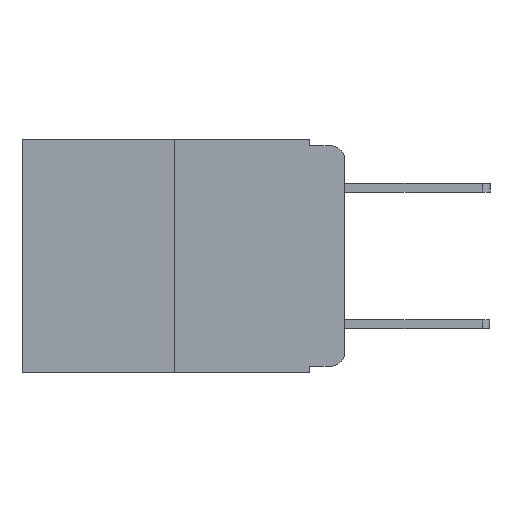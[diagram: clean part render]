
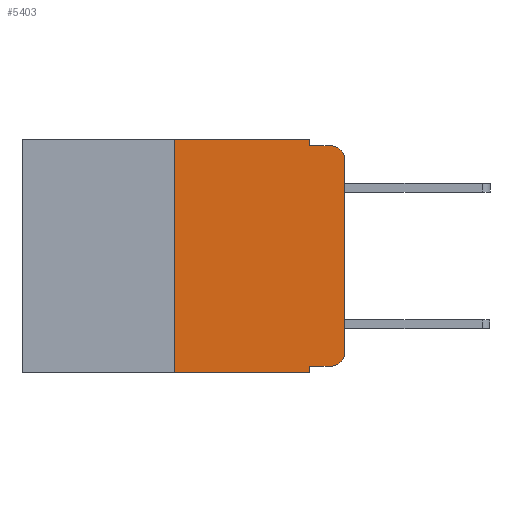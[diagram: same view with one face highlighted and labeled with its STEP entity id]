
A CAD part, left-side view. The second image highlights one B-rep face of the part: STEP entity #5403.
In plain terms, the highlighted planar face has unit normal (-1, 0, 0).
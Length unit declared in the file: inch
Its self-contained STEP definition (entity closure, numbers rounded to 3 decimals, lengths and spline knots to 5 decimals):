
#207 = VERTEX_POINT ( 'NONE', #18770 ) ;
#212 = DIRECTION ( 'NONE',  ( -1., 0., 0. ) ) ;
#791 = VECTOR ( 'NONE', #21845, 39.37008 ) ;
#1542 = VERTEX_POINT ( 'NONE', #19385 ) ;
#1869 = CARTESIAN_POINT ( 'NONE',  ( 0., 0., -0.03 ) ) ;
#1875 = DIRECTION ( 'NONE',  ( 0., 0., -1. ) ) ;
#2363 = VERTEX_POINT ( 'NONE', #11058 ) ;
#2565 = VECTOR ( 'NONE', #14616, 39.37008 ) ;
#2620 = EDGE_CURVE ( 'NONE', #9207, #5391, #18414, .T. ) ;
#2834 = DIRECTION ( 'NONE',  ( -1., 0., 0. ) ) ;
#3682 = DIRECTION ( 'NONE',  ( 0., 0., 1. ) ) ;
#3754 = VERTEX_POINT ( 'NONE', #19878 ) ;
#3795 = CARTESIAN_POINT ( 'NONE',  ( 0., 0.473, -0.343 ) ) ;
#4409 = VERTEX_POINT ( 'NONE', #1869 ) ;
#4679 = DIRECTION ( 'NONE',  ( 1., 0., 0. ) ) ;
#4725 = EDGE_CURVE ( 'NONE', #4409, #1542, #7290, .T. ) ;
#4812 = VECTOR ( 'NONE', #3682, 39.37008 ) ;
#5391 = VERTEX_POINT ( 'NONE', #15419 ) ;
#5403 = ADVANCED_FACE ( 'NONE', ( #17141 ), #22650, .F. ) ;
#5449 = AXIS2_PLACEMENT_3D ( 'NONE', #11180, #212, #12978 ) ;
#5974 = VERTEX_POINT ( 'NONE', #20781 ) ;
#6327 = LINE ( 'NONE', #3795, #2565 ) ;
#6344 = ORIENTED_EDGE ( 'NONE', *, *, #19648, .F. ) ;
#6492 = DIRECTION ( 'NONE',  ( 0., -1., 0. ) ) ;
#6528 = LINE ( 'NONE', #18198, #4812 ) ;
#6679 = ORIENTED_EDGE ( 'NONE', *, *, #6834, .T. ) ;
#6746 = VERTEX_POINT ( 'NONE', #15909 ) ;
#6834 = EDGE_CURVE ( 'NONE', #5974, #5391, #6327, .T. ) ;
#6891 = CARTESIAN_POINT ( 'NONE',  ( 0., 0.051, -0.333 ) ) ;
#6911 = VECTOR ( 'NONE', #1875, 39.37008 ) ;
#7230 = VECTOR ( 'NONE', #8266, 39.37008 ) ;
#7290 = CIRCLE ( 'NONE', #8302, 0.02 ) ;
#7409 = CIRCLE ( 'NONE', #5449, 0.02 ) ;
#7461 = EDGE_CURVE ( 'NONE', #207, #2363, #21291, .T. ) ;
#8266 = DIRECTION ( 'NONE',  ( 0., -1., 0. ) ) ;
#8302 = AXIS2_PLACEMENT_3D ( 'NONE', #13658, #2834, #15533 ) ;
#8913 = CARTESIAN_POINT ( 'NONE',  ( 0., 0.02, -0.333 ) ) ;
#9089 = EDGE_CURVE ( 'NONE', #9207, #21741, #16703, .T. ) ;
#9207 = VERTEX_POINT ( 'NONE', #6891 ) ;
#9549 = ORIENTED_EDGE ( 'NONE', *, *, #2620, .F. ) ;
#9586 = CARTESIAN_POINT ( 'NONE',  ( 0., 0.473, 0. ) ) ;
#10154 = EDGE_LOOP ( 'NONE', ( #18656, #12806, #12876, #14495, #6344, #20936, #6679, #9549, #19406, #23187 ) ) ;
#11058 = CARTESIAN_POINT ( 'NONE',  ( 0., 0.051, -0.01 ) ) ;
#11180 = CARTESIAN_POINT ( 'NONE',  ( 0., 0.02, -0.313 ) ) ;
#11635 = LINE ( 'NONE', #14508, #791 ) ;
#12806 = ORIENTED_EDGE ( 'NONE', *, *, #4725, .T. ) ;
#12876 = ORIENTED_EDGE ( 'NONE', *, *, #14815, .F. ) ;
#12978 = DIRECTION ( 'NONE',  ( 0., 0., -1. ) ) ;
#13557 = CARTESIAN_POINT ( 'NONE',  ( 0., 0.473, 0. ) ) ;
#13611 = CARTESIAN_POINT ( 'NONE',  ( 0., 0.051, -0.333 ) ) ;
#13658 = CARTESIAN_POINT ( 'NONE',  ( 0., 0.02, -0.03 ) ) ;
#14495 = ORIENTED_EDGE ( 'NONE', *, *, #7461, .F. ) ;
#14508 = CARTESIAN_POINT ( 'NONE',  ( 0., 0., 0. ) ) ;
#14616 = DIRECTION ( 'NONE',  ( 0., -1., 0. ) ) ;
#14815 = EDGE_CURVE ( 'NONE', #2363, #1542, #16263, .T. ) ;
#15419 = CARTESIAN_POINT ( 'NONE',  ( 0., 0.051, -0.343 ) ) ;
#15533 = DIRECTION ( 'NONE',  ( 0., 0., -1. ) ) ;
#15864 = AXIS2_PLACEMENT_3D ( 'NONE', #13557, #4679, #17358 ) ;
#15909 = CARTESIAN_POINT ( 'NONE',  ( 0., 0., -0.313 ) ) ;
#16247 = EDGE_CURVE ( 'NONE', #6746, #4409, #11635, .T. ) ;
#16263 = LINE ( 'NONE', #19087, #7230 ) ;
#16703 = LINE ( 'NONE', #13611, #20922 ) ;
#16864 = DIRECTION ( 'NONE',  ( 0., -1., 0. ) ) ;
#17141 = FACE_OUTER_BOUND ( 'NONE', #10154, .T. ) ;
#17358 = DIRECTION ( 'NONE',  ( 0., 0., -1. ) ) ;
#17581 = EDGE_CURVE ( 'NONE', #21741, #6746, #7409, .T. ) ;
#18198 = CARTESIAN_POINT ( 'NONE',  ( 0., 0.25, 0. ) ) ;
#18414 = LINE ( 'NONE', #20811, #22583 ) ;
#18594 = VECTOR ( 'NONE', #16864, 39.37008 ) ;
#18656 = ORIENTED_EDGE ( 'NONE', *, *, #16247, .T. ) ;
#18770 = CARTESIAN_POINT ( 'NONE',  ( 0., 0.051, 0. ) ) ;
#19087 = CARTESIAN_POINT ( 'NONE',  ( 0., 0.051, -0.01 ) ) ;
#19385 = CARTESIAN_POINT ( 'NONE',  ( 0., 0.02, -0.01 ) ) ;
#19406 = ORIENTED_EDGE ( 'NONE', *, *, #9089, .T. ) ;
#19648 = EDGE_CURVE ( 'NONE', #3754, #207, #23319, .T. ) ;
#19878 = CARTESIAN_POINT ( 'NONE',  ( 0., 0.25, 0. ) ) ;
#20781 = CARTESIAN_POINT ( 'NONE',  ( 0., 0.25, -0.343 ) ) ;
#20811 = CARTESIAN_POINT ( 'NONE',  ( 0., 0.051, 0. ) ) ;
#20922 = VECTOR ( 'NONE', #6492, 39.37008 ) ;
#20936 = ORIENTED_EDGE ( 'NONE', *, *, #22511, .F. ) ;
#21291 = LINE ( 'NONE', #23540, #6911 ) ;
#21741 = VERTEX_POINT ( 'NONE', #8913 ) ;
#21845 = DIRECTION ( 'NONE',  ( 0., 0., 1. ) ) ;
#22511 = EDGE_CURVE ( 'NONE', #5974, #3754, #6528, .T. ) ;
#22581 = DIRECTION ( 'NONE',  ( 0., 0., -1. ) ) ;
#22583 = VECTOR ( 'NONE', #22581, 39.37008 ) ;
#22650 = PLANE ( 'NONE',  #15864 ) ;
#23187 = ORIENTED_EDGE ( 'NONE', *, *, #17581, .T. ) ;
#23319 = LINE ( 'NONE', #9586, #18594 ) ;
#23540 = CARTESIAN_POINT ( 'NONE',  ( 0., 0.051, 0. ) ) ;
